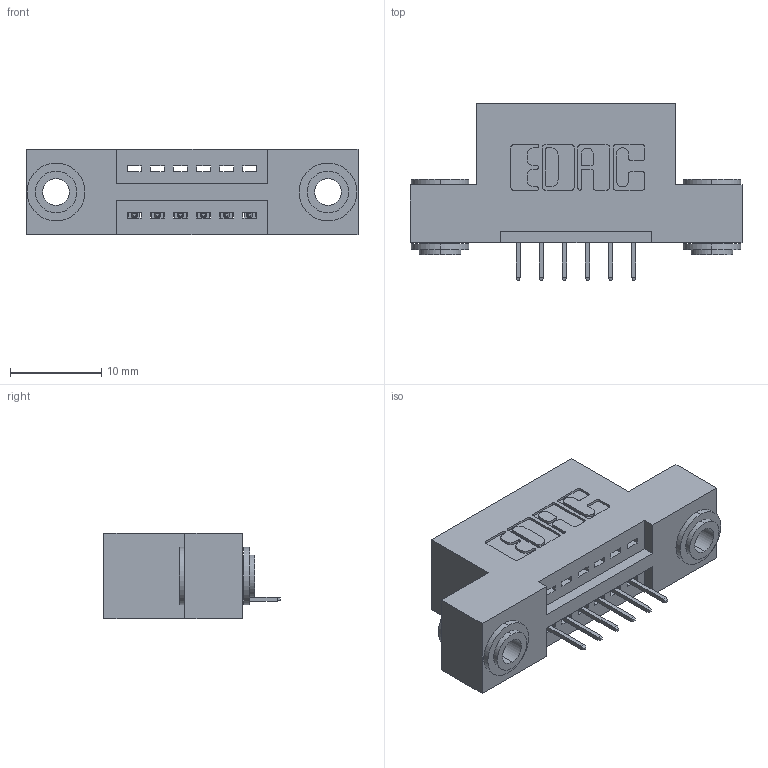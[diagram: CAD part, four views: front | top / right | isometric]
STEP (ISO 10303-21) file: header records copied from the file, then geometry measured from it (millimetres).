
FILE_DESCRIPTION (( 'STEP AP203' ), '1' );
FILE_NAME ('395-006-524-103.STEP', '2019-10-15T15:43:19', ( '' ), ( '' ), 'SwSTEP 2.0', 'SolidWorks 2016', '' );
FILE_SCHEMA (( 'CONFIG_CONTROL_DESIGN' ));
Length unit declared in the file: inch
Products named in the file (4): 395-006-524-103; 345 Part_Flush Mounting Lugs - 0.156 Dia-TH; 345-292-001_345-293-124; 345-250-002_345-250-002-102
Assembly tree (9 placements, depth 2):
  395-006-524-103
    345 Part_Flush Mounting Lugs - 0.156 Dia-TH
    345-292-001_345-293-124  x6
    345-250-002_345-250-002-102  x2
Bounding box: 36.45 x 19.35 x 9.4 mm (x, y, z)
Volume: 3162.8 mm3; surface area: 3852.4 mm2
Topology: 9 solids, 9 shells, 536 faces, 1497 edges, 970 vertices
Faces by surface type: plane 366, cylinder 162, cone 8
Entity records: 10086 total; most frequent: CARTESIAN_POINT 1725, ORIENTED_EDGE 1658, DIRECTION 1591, EDGE_CURVE 829, VECTOR 653, LINE 653, VERTEX_POINT 546, AXIS2_PLACEMENT_3D 469
